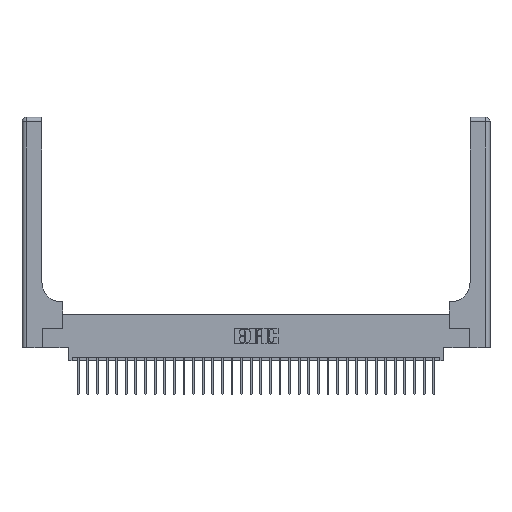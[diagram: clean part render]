
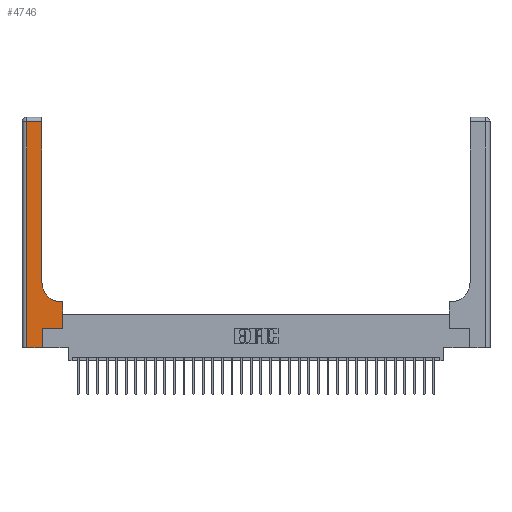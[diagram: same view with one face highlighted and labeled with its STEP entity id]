
A CAD part, top view. The second image highlights one B-rep face of the part: STEP entity #4746.
In plain terms, the highlighted planar face has unit normal (0, 0, 1).
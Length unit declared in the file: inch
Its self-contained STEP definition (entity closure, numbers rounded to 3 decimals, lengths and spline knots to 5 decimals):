
#974 = LINE ( 'NONE', #13195, #25502 ) ;
#1350 = DIRECTION ( 'NONE',  ( -1., 0., 0. ) ) ;
#1409 = DIRECTION ( 'NONE',  ( -1., 0., 0. ) ) ;
#1824 = AXIS2_PLACEMENT_3D ( 'NONE', #27194, #13024, #29569 ) ;
#2421 = CARTESIAN_POINT ( 'NONE',  ( 0.265, 0.25, 0.37 ) ) ;
#2423 = CARTESIAN_POINT ( 'NONE',  ( 0.26, 2.94, 0.37 ) ) ;
#2668 = PLANE ( 'NONE',  #25040 ) ;
#3525 = DIRECTION ( 'NONE',  ( 0., 1., 0. ) ) ;
#4715 = ORIENTED_EDGE ( 'NONE', *, *, #22443, .T. ) ;
#4746 = ADVANCED_FACE ( 'NONE', ( #29742 ), #2668, .F. ) ;
#4776 = VECTOR ( 'NONE', #30671, 39.37008 ) ;
#5080 = DIRECTION ( 'NONE',  ( 0., 0., -1. ) ) ;
#5185 = LINE ( 'NONE', #24081, #17043 ) ;
#5919 = VERTEX_POINT ( 'NONE', #9624 ) ;
#6101 = CARTESIAN_POINT ( 'NONE',  ( 0.26, 0.6, 0.37 ) ) ;
#6435 = VECTOR ( 'NONE', #3525, 39.37008 ) ;
#6703 = DIRECTION ( 'NONE',  ( 0., 1., 0. ) ) ;
#7092 = LINE ( 'NONE', #27717, #23824 ) ;
#7404 = VERTEX_POINT ( 'NONE', #20025 ) ;
#8302 = ORIENTED_EDGE ( 'NONE', *, *, #27136, .T. ) ;
#8824 = VECTOR ( 'NONE', #9220, 39.37008 ) ;
#9220 = DIRECTION ( 'NONE',  ( 0., -1., 0. ) ) ;
#9583 = LINE ( 'NONE', #13902, #8824 ) ;
#9624 = CARTESIAN_POINT ( 'NONE',  ( 0.528, 0.6, 0.37 ) ) ;
#9696 = ORIENTED_EDGE ( 'NONE', *, *, #11535, .T. ) ;
#9892 = LINE ( 'NONE', #20956, #27287 ) ;
#10582 = VERTEX_POINT ( 'NONE', #20888 ) ;
#11535 = EDGE_CURVE ( 'NONE', #5919, #18580, #28734, .T. ) ;
#11857 = LINE ( 'NONE', #25974, #4776 ) ;
#12255 = DIRECTION ( 'NONE',  ( 0., 1., 0. ) ) ;
#13024 = DIRECTION ( 'NONE',  ( 0., 0., -1. ) ) ;
#13195 = CARTESIAN_POINT ( 'NONE',  ( 0., 2.94, 0.37 ) ) ;
#13379 = VERTEX_POINT ( 'NONE', #18730 ) ;
#13499 = LINE ( 'NONE', #27153, #6435 ) ;
#13591 = ORIENTED_EDGE ( 'NONE', *, *, #24744, .T. ) ;
#13902 = CARTESIAN_POINT ( 'NONE',  ( 0.06, 3., 0.37 ) ) ;
#14221 = CIRCLE ( 'NONE', #1824, 0.25 ) ;
#14511 = CARTESIAN_POINT ( 'NONE',  ( 0., 3., 0.37 ) ) ;
#14965 = ORIENTED_EDGE ( 'NONE', *, *, #21691, .T. ) ;
#15134 = CARTESIAN_POINT ( 'NONE',  ( 0.06, 2.94, 0.37 ) ) ;
#15872 = VERTEX_POINT ( 'NONE', #26567 ) ;
#16811 = EDGE_CURVE ( 'NONE', #10582, #13379, #7092, .T. ) ;
#17043 = VECTOR ( 'NONE', #12255, 39.37008 ) ;
#18203 = ORIENTED_EDGE ( 'NONE', *, *, #20400, .T. ) ;
#18289 = EDGE_CURVE ( 'NONE', #21369, #15872, #11857, .T. ) ;
#18580 = VERTEX_POINT ( 'NONE', #29330 ) ;
#18730 = CARTESIAN_POINT ( 'NONE',  ( 0.265, 0., 0.37 ) ) ;
#18843 = EDGE_CURVE ( 'NONE', #20962, #10582, #9583, .T. ) ;
#19408 = ORIENTED_EDGE ( 'NONE', *, *, #16811, .T. ) ;
#20025 = CARTESIAN_POINT ( 'NONE',  ( 0.26, 0.85, 0.37 ) ) ;
#20400 = EDGE_CURVE ( 'NONE', #25384, #20962, #974, .T. ) ;
#20888 = CARTESIAN_POINT ( 'NONE',  ( 0.06, 0., 0.37 ) ) ;
#20956 = CARTESIAN_POINT ( 'NONE',  ( 0.528, 0.25, 0.37 ) ) ;
#20962 = VERTEX_POINT ( 'NONE', #15134 ) ;
#21044 = EDGE_LOOP ( 'NONE', ( #4715, #18203, #22127, #19408, #13591, #29246, #8302, #9696, #14965 ) ) ;
#21369 = VERTEX_POINT ( 'NONE', #2421 ) ;
#21689 = DIRECTION ( 'NONE',  ( -1., 0., 0. ) ) ;
#21691 = EDGE_CURVE ( 'NONE', #18580, #7404, #14221, .T. ) ;
#21734 = VECTOR ( 'NONE', #1409, 39.37008 ) ;
#22127 = ORIENTED_EDGE ( 'NONE', *, *, #18843, .T. ) ;
#22443 = EDGE_CURVE ( 'NONE', #7404, #25384, #13499, .T. ) ;
#23824 = VECTOR ( 'NONE', #25392, 39.37008 ) ;
#24081 = CARTESIAN_POINT ( 'NONE',  ( 0.265, 0., 0.37 ) ) ;
#24744 = EDGE_CURVE ( 'NONE', #13379, #21369, #5185, .T. ) ;
#25040 = AXIS2_PLACEMENT_3D ( 'NONE', #14511, #5080, #21689 ) ;
#25384 = VERTEX_POINT ( 'NONE', #2423 ) ;
#25392 = DIRECTION ( 'NONE',  ( 1., 0., 0. ) ) ;
#25502 = VECTOR ( 'NONE', #1350, 39.37008 ) ;
#25974 = CARTESIAN_POINT ( 'NONE',  ( 0.265, 0.25, 0.37 ) ) ;
#26567 = CARTESIAN_POINT ( 'NONE',  ( 0.528, 0.25, 0.37 ) ) ;
#27136 = EDGE_CURVE ( 'NONE', #15872, #5919, #9892, .T. ) ;
#27153 = CARTESIAN_POINT ( 'NONE',  ( 0.26, 3., 0.37 ) ) ;
#27194 = CARTESIAN_POINT ( 'NONE',  ( 0.51, 0.85, 0.37 ) ) ;
#27287 = VECTOR ( 'NONE', #6703, 39.37008 ) ;
#27717 = CARTESIAN_POINT ( 'NONE',  ( 0., 0., 0.37 ) ) ;
#28734 = LINE ( 'NONE', #6101, #21734 ) ;
#29246 = ORIENTED_EDGE ( 'NONE', *, *, #18289, .T. ) ;
#29330 = CARTESIAN_POINT ( 'NONE',  ( 0.51, 0.6, 0.37 ) ) ;
#29569 = DIRECTION ( 'NONE',  ( 1., 0., 0. ) ) ;
#29742 = FACE_OUTER_BOUND ( 'NONE', #21044, .T. ) ;
#30671 = DIRECTION ( 'NONE',  ( 1., 0., 0. ) ) ;
